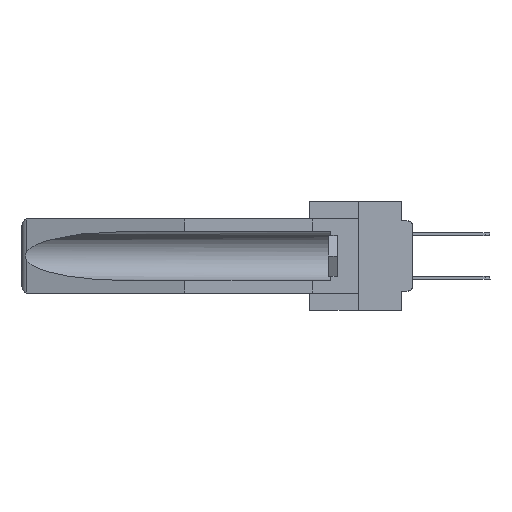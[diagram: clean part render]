
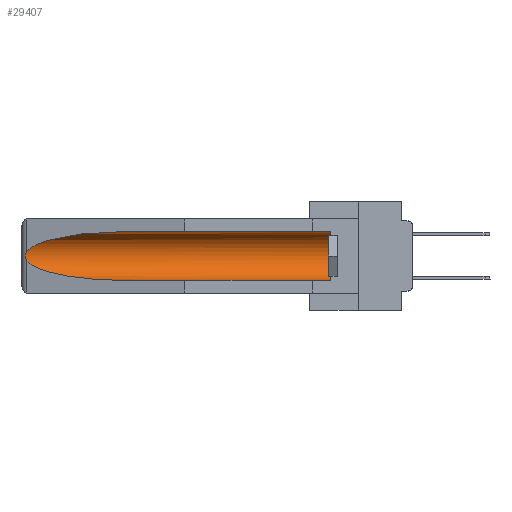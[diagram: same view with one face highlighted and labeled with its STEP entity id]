
A CAD part, left-side view. The second image highlights one B-rep face of the part: STEP entity #29407.
In plain terms, the highlighted cylindrical face has radius 2.857 mm (diameter 5.715 mm), a partial arc.
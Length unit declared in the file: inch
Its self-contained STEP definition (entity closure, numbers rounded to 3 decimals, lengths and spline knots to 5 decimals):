
#1175 =( BOUNDED_CURVE ( )  B_SPLINE_CURVE ( 3, ( #24518, #18465, #10136, #1561 ),
 .UNSPECIFIED., .F., .T. ) 
 B_SPLINE_CURVE_WITH_KNOTS ( ( 4, 4 ),
 ( 0.1948, 1.5708 ),
 .UNSPECIFIED. ) 
 CURVE ( )  GEOMETRIC_REPRESENTATION_ITEM ( )  RATIONAL_B_SPLINE_CURVE ( ( 1., 0.848, 0.848, 1. ) ) 
 REPRESENTATION_ITEM ( '' )  );
#1411 = CARTESIAN_POINT ( 'NONE',  ( 0.155, 0.126, -0.059 ) ) ;
#1561 = CARTESIAN_POINT ( 'NONE',  ( 0.155, 1.07973, -0.284 ) ) ;
#2154 = CARTESIAN_POINT ( 'NONE',  ( 0.155, 1.07973, -0.059 ) ) ;
#2332 = CARTESIAN_POINT ( 'NONE',  ( 0.155, -0.30754, -0.059 ) ) ;
#3459 = VERTEX_POINT ( 'NONE', #35528 ) ;
#3791 = ORIENTED_EDGE ( 'NONE', *, *, #24290, .T. ) ;
#3857 = CIRCLE ( 'NONE', #20830, 0.1125 ) ;
#4069 = CARTESIAN_POINT ( 'NONE',  ( 0.26537, 1.52718, -0.14972 ) ) ;
#5150 = VECTOR ( 'NONE', #18993, 39.37008 ) ;
#6492 = EDGE_CURVE ( 'NONE', #9389, #3459, #16778, .T. ) ;
#7794 = B_SPLINE_CURVE_WITH_KNOTS ( 'NONE', 3,
 ( #4069, #21536, #35740, #12818, #18684, #30234, #35552, #15859, #9603, #27382 ),
 .UNSPECIFIED., .F., .F.,
 ( 4, 2, 2, 2, 4 ),
 ( 0., 0.00029, 0.00058, 0.00087, 0.00117 ),
 .UNSPECIFIED. ) ;
#8240 = DIRECTION ( 'NONE',  ( 0., 1., 0. ) ) ;
#8266 = DIRECTION ( 'NONE',  ( 0., 1., 0. ) ) ;
#8469 = VERTEX_POINT ( 'NONE', #35648 ) ;
#9389 = VERTEX_POINT ( 'NONE', #1411 ) ;
#9603 = CARTESIAN_POINT ( 'NONE',  ( 0.26597, 1.5296, -0.19026 ) ) ;
#9822 = DIRECTION ( 'NONE',  ( 0., -1., 0. ) ) ;
#10136 = CARTESIAN_POINT ( 'NONE',  ( 0.21114, 1.30732, -0.284 ) ) ;
#10138 = EDGE_CURVE ( 'NONE', #3459, #23507, #15289, .T. ) ;
#12818 = CARTESIAN_POINT ( 'NONE',  ( 0.2673, 1.5327, -0.16383 ) ) ;
#13700 = EDGE_CURVE ( 'NONE', #15946, #9389, #3857, .T. ) ;
#13732 = VECTOR ( 'NONE', #8240, 39.37008 ) ;
#13746 = CARTESIAN_POINT ( 'NONE',  ( 0.21114, 1.30732, -0.059 ) ) ;
#15289 =( BOUNDED_CURVE ( )  B_SPLINE_CURVE ( 3, ( #2154, #13746, #25290, #36857 ),
 .UNSPECIFIED., .F., .T. ) 
 B_SPLINE_CURVE_WITH_KNOTS ( ( 4, 4 ),
 ( 4.71239, 6.08839 ),
 .UNSPECIFIED. ) 
 CURVE ( )  GEOMETRIC_REPRESENTATION_ITEM ( )  RATIONAL_B_SPLINE_CURVE ( ( 1., 0.848, 0.848, 1. ) ) 
 REPRESENTATION_ITEM ( '' )  );
#15859 = CARTESIAN_POINT ( 'NONE',  ( 0.26655, 1.53094, -0.18657 ) ) ;
#15946 = VERTEX_POINT ( 'NONE', #16714 ) ;
#16433 = CARTESIAN_POINT ( 'NONE',  ( 0.155, -0.30754, -0.1715 ) ) ;
#16714 = CARTESIAN_POINT ( 'NONE',  ( 0.155, 0.126, -0.284 ) ) ;
#16731 = ORIENTED_EDGE ( 'NONE', *, *, #13700, .T. ) ;
#16778 = LINE ( 'NONE', #2332, #13732 ) ;
#17619 = EDGE_LOOP ( 'NONE', ( #35549, #3791, #35805, #30427, #16731, #34275 ) ) ;
#18465 = CARTESIAN_POINT ( 'NONE',  ( 0.25451, 1.48313, -0.24835 ) ) ;
#18684 = CARTESIAN_POINT ( 'NONE',  ( 0.2675, 1.53308, -0.16763 ) ) ;
#18993 = DIRECTION ( 'NONE',  ( 0., 1., 0. ) ) ;
#19007 = CARTESIAN_POINT ( 'NONE',  ( 0.26537, 1.52718, -0.14972 ) ) ;
#19263 = FACE_OUTER_BOUND ( 'NONE', #17619, .T. ) ;
#20830 = AXIS2_PLACEMENT_3D ( 'NONE', #32928, #9822, #26864 ) ;
#21536 = CARTESIAN_POINT ( 'NONE',  ( 0.26597, 1.52961, -0.15275 ) ) ;
#21705 = EDGE_CURVE ( 'NONE', #8469, #25805, #1175, .T. ) ;
#22296 = DIRECTION ( 'NONE',  ( 0., 0., 1. ) ) ;
#23507 = VERTEX_POINT ( 'NONE', #19007 ) ;
#24290 = EDGE_CURVE ( 'NONE', #23507, #8469, #7794, .T. ) ;
#24518 = CARTESIAN_POINT ( 'NONE',  ( 0.26537, 1.52718, -0.19328 ) ) ;
#25290 = CARTESIAN_POINT ( 'NONE',  ( 0.25451, 1.48313, -0.09465 ) ) ;
#25805 = VERTEX_POINT ( 'NONE', #26426 ) ;
#26426 = CARTESIAN_POINT ( 'NONE',  ( 0.155, 1.07973, -0.284 ) ) ;
#26864 = DIRECTION ( 'NONE',  ( 0., 0., 1. ) ) ;
#27128 = CARTESIAN_POINT ( 'NONE',  ( 0.155, -0.30754, -0.284 ) ) ;
#27382 = CARTESIAN_POINT ( 'NONE',  ( 0.26537, 1.52718, -0.19328 ) ) ;
#27886 = LINE ( 'NONE', #27128, #5150 ) ;
#29407 = ADVANCED_FACE ( 'NONE', ( #19263 ), #37065, .F. ) ;
#30234 = CARTESIAN_POINT ( 'NONE',  ( 0.2675, 1.53308, -0.17534 ) ) ;
#30427 = ORIENTED_EDGE ( 'NONE', *, *, #34407, .F. ) ;
#32608 = AXIS2_PLACEMENT_3D ( 'NONE', #16433, #8266, #22296 ) ;
#32928 = CARTESIAN_POINT ( 'NONE',  ( 0.155, 0.126, -0.1715 ) ) ;
#34275 = ORIENTED_EDGE ( 'NONE', *, *, #6492, .T. ) ;
#34407 = EDGE_CURVE ( 'NONE', #15946, #25805, #27886, .T. ) ;
#35528 = CARTESIAN_POINT ( 'NONE',  ( 0.155, 1.07973, -0.059 ) ) ;
#35549 = ORIENTED_EDGE ( 'NONE', *, *, #10138, .T. ) ;
#35552 = CARTESIAN_POINT ( 'NONE',  ( 0.2673, 1.53269, -0.17917 ) ) ;
#35648 = CARTESIAN_POINT ( 'NONE',  ( 0.26537, 1.52718, -0.19328 ) ) ;
#35740 = CARTESIAN_POINT ( 'NONE',  ( 0.26654, 1.53092, -0.15636 ) ) ;
#35805 = ORIENTED_EDGE ( 'NONE', *, *, #21705, .T. ) ;
#36857 = CARTESIAN_POINT ( 'NONE',  ( 0.26537, 1.52718, -0.14972 ) ) ;
#37065 = CYLINDRICAL_SURFACE ( 'NONE', #32608, 0.1125 ) ;
